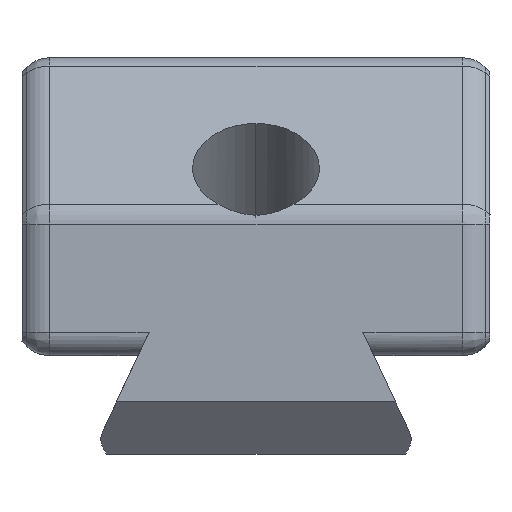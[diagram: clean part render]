
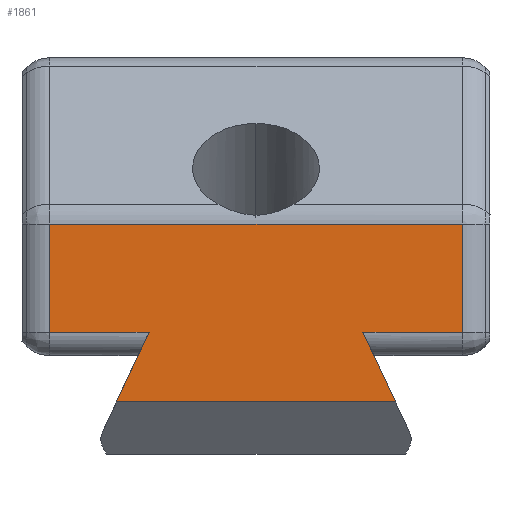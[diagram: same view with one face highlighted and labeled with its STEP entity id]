
A CAD part, left-side view. The second image highlights one B-rep face of the part: STEP entity #1861.
In plain terms, the highlighted planar face has unit normal (-1, 0, 0).
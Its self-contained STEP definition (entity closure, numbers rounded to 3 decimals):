
#41=PLANE('',#2060);
#113=LINE('',#2879,#262);
#138=LINE('',#3029,#287);
#164=LINE('',#3229,#313);
#191=LINE('',#3410,#340);
#192=LINE('',#3414,#341);
#193=LINE('',#3416,#342);
#194=LINE('',#3417,#343);
#195=LINE('',#3418,#344);
#262=VECTOR('',#2197,10.);
#287=VECTOR('',#2290,10.);
#313=VECTOR('',#2380,10.);
#340=VECTOR('',#2493,10.);
#341=VECTOR('',#2498,10.);
#342=VECTOR('',#2499,10.);
#343=VECTOR('',#2500,10.);
#344=VECTOR('',#2501,10.);
#511=FACE_OUTER_BOUND('',#632,.T.);
#632=EDGE_LOOP('',(#1533,#1534,#1535,#1536,#1537,#1538,#1539,#1540));
#823=VERTEX_POINT('',#2872);
#825=VERTEX_POINT('',#2878);
#851=VERTEX_POINT('',#3027);
#883=VERTEX_POINT('',#3222);
#885=VERTEX_POINT('',#3228);
#913=VERTEX_POINT('',#3409);
#914=VERTEX_POINT('',#3413);
#915=VERTEX_POINT('',#3415);
#991=EDGE_CURVE('',#823,#825,#113,.T.);
#1039=EDGE_CURVE('',#851,#823,#138,.T.);
#1089=EDGE_CURVE('',#883,#885,#164,.T.);
#1144=EDGE_CURVE('',#885,#913,#191,.T.);
#1146=EDGE_CURVE('',#851,#914,#192,.T.);
#1147=EDGE_CURVE('',#914,#915,#193,.T.);
#1148=EDGE_CURVE('',#915,#913,#194,.F.);
#1149=EDGE_CURVE('',#825,#883,#195,.T.);
#1533=ORIENTED_EDGE('',*,*,#991,.F.);
#1534=ORIENTED_EDGE('',*,*,#1039,.F.);
#1535=ORIENTED_EDGE('',*,*,#1146,.T.);
#1536=ORIENTED_EDGE('',*,*,#1147,.T.);
#1537=ORIENTED_EDGE('',*,*,#1148,.T.);
#1538=ORIENTED_EDGE('',*,*,#1144,.F.);
#1539=ORIENTED_EDGE('',*,*,#1089,.F.);
#1540=ORIENTED_EDGE('',*,*,#1149,.F.);
#1861=ADVANCED_FACE('',(#511),#41,.T.);
#2060=AXIS2_PLACEMENT_3D('',#3412,#2496,#2497);
#2197=DIRECTION('',(0.,0.,1.));
#2290=DIRECTION('',(0.,1.,0.));
#2380=DIRECTION('',(0.,0.,-1.));
#2493=DIRECTION('',(0.,1.,0.));
#2496=DIRECTION('center_axis',(-1.,0.,0.));
#2497=DIRECTION('ref_axis',(0.,0.,1.));
#2498=DIRECTION('',(0.,0.423,-0.906));
#2499=DIRECTION('',(0.,-1.,0.));
#2500=DIRECTION('',(0.,-0.423,-0.906));
#2501=DIRECTION('',(0.,-1.,0.));
#2872=CARTESIAN_POINT('',(-9.4,7.169,2.6));
#2878=CARTESIAN_POINT('',(-9.4,7.169,4.905));
#2879=CARTESIAN_POINT('',(-9.4,7.169,1.079));
#3027=CARTESIAN_POINT('',(-9.4,5.052,2.6));
#3029=CARTESIAN_POINT('',(-9.4,15.389,2.6));
#3222=CARTESIAN_POINT('',(-9.4,-1.624,4.905));
#3228=CARTESIAN_POINT('',(-9.4,-1.624,2.6));
#3229=CARTESIAN_POINT('',(-9.4,-1.624,1.079));
#3409=CARTESIAN_POINT('',(-9.4,0.493,2.6));
#3410=CARTESIAN_POINT('',(-9.4,-12.578,2.6));
#3412=CARTESIAN_POINT('Origin',(-9.4,0.039,0.281));
#3413=CARTESIAN_POINT('',(-9.4,5.746,1.112));
#3414=CARTESIAN_POINT('',(-9.4,5.108,2.479));
#3415=CARTESIAN_POINT('',(-9.4,-0.202,1.112));
#3416=CARTESIAN_POINT('',(-9.4,-2.211,1.112));
#3417=CARTESIAN_POINT('',(-9.4,-0.052,1.431));
#3418=CARTESIAN_POINT('',(-9.4,7.714,4.905));
